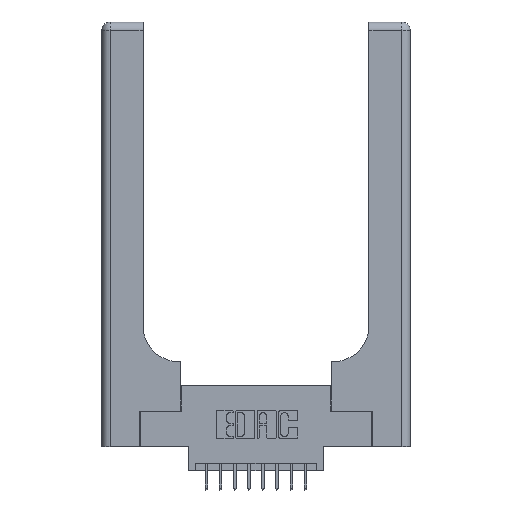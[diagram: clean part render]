
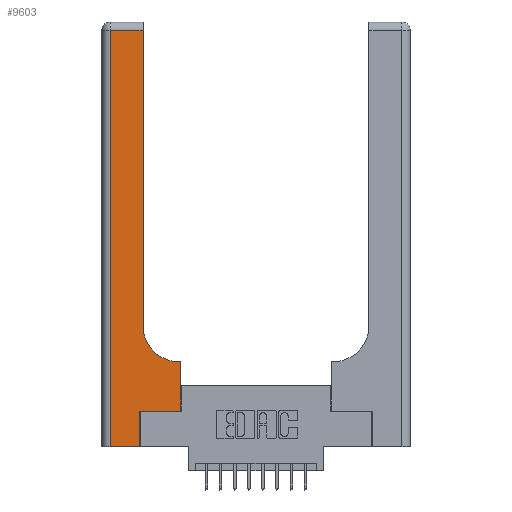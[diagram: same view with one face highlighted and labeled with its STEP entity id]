
A CAD part, top view. The second image highlights one B-rep face of the part: STEP entity #9603.
In plain terms, the highlighted planar face has unit normal (0, 0, 1).
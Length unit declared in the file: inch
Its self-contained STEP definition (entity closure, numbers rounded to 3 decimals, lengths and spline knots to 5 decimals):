
#223 = CARTESIAN_POINT ( 'NONE',  ( 0.2915, 2.94, 0.37 ) ) ;
#369 = DIRECTION ( 'NONE',  ( -1., 0., 0. ) ) ;
#524 = VERTEX_POINT ( 'NONE', #11892 ) ;
#541 = CARTESIAN_POINT ( 'NONE',  ( 0.2915, 3., 0.37 ) ) ;
#548 = CARTESIAN_POINT ( 'NONE',  ( 0.5415, 0.6, 0.37 ) ) ;
#1039 = ORIENTED_EDGE ( 'NONE', *, *, #4788, .T. ) ;
#1238 = VERTEX_POINT ( 'NONE', #223 ) ;
#1439 = CARTESIAN_POINT ( 'NONE',  ( 0., 2.94, 0.37 ) ) ;
#1464 = VERTEX_POINT ( 'NONE', #9798 ) ;
#1492 = AXIS2_PLACEMENT_3D ( 'NONE', #4526, #3270, #8075 ) ;
#1520 = LINE ( 'NONE', #5147, #5695 ) ;
#1839 = DIRECTION ( 'NONE',  ( -1., 0., 0. ) ) ;
#2392 = CARTESIAN_POINT ( 'NONE',  ( 0.06, 3., 0.37 ) ) ;
#2693 = DIRECTION ( 'NONE',  ( 0., 1., 0. ) ) ;
#2782 = ORIENTED_EDGE ( 'NONE', *, *, #4638, .T. ) ;
#2854 = VECTOR ( 'NONE', #6814, 39.37008 ) ;
#2928 = EDGE_CURVE ( 'NONE', #14129, #7966, #8968, .T. ) ;
#3190 = ORIENTED_EDGE ( 'NONE', *, *, #11571, .T. ) ;
#3215 = CARTESIAN_POINT ( 'NONE',  ( 0.269, 0.25, 0.37 ) ) ;
#3270 = DIRECTION ( 'NONE',  ( 0., 0., -1. ) ) ;
#3333 = ORIENTED_EDGE ( 'NONE', *, *, #12594, .T. ) ;
#3641 = EDGE_CURVE ( 'NONE', #1464, #1238, #4170, .T. ) ;
#3758 = CARTESIAN_POINT ( 'NONE',  ( 0.06, 2.94, 0.37 ) ) ;
#3923 = DIRECTION ( 'NONE',  ( -1., 0., 0. ) ) ;
#3999 = LINE ( 'NONE', #1439, #8890 ) ;
#4091 = CARTESIAN_POINT ( 'NONE',  ( 0.5585, 0.25, 0.37 ) ) ;
#4170 = LINE ( 'NONE', #541, #2854 ) ;
#4375 = CARTESIAN_POINT ( 'NONE',  ( 0.2915, 0.6, 0.37 ) ) ;
#4526 = CARTESIAN_POINT ( 'NONE',  ( 0.5415, 0.85, 0.37 ) ) ;
#4638 = EDGE_CURVE ( 'NONE', #10587, #1464, #10687, .T. ) ;
#4788 = EDGE_CURVE ( 'NONE', #15044, #14129, #1520, .T. ) ;
#4975 = CARTESIAN_POINT ( 'NONE',  ( 0.269, 0., 0.37 ) ) ;
#5147 = CARTESIAN_POINT ( 'NONE',  ( 0., 0., 0.37 ) ) ;
#5411 = VECTOR ( 'NONE', #11277, 39.37008 ) ;
#5695 = VECTOR ( 'NONE', #15281, 39.37008 ) ;
#6079 = VERTEX_POINT ( 'NONE', #3758 ) ;
#6111 = CARTESIAN_POINT ( 'NONE',  ( 0.269, 0.25, 0.37 ) ) ;
#6311 = CARTESIAN_POINT ( 'NONE',  ( 0.5585, 0.25, 0.37 ) ) ;
#6644 = FACE_OUTER_BOUND ( 'NONE', #7643, .T. ) ;
#6814 = DIRECTION ( 'NONE',  ( 0., 1., 0. ) ) ;
#7643 = EDGE_LOOP ( 'NONE', ( #9499, #9188, #3333, #1039, #12235, #13364, #3190, #9323, #2782 ) ) ;
#7966 = VERTEX_POINT ( 'NONE', #6111 ) ;
#7977 = AXIS2_PLACEMENT_3D ( 'NONE', #12908, #10178, #369 ) ;
#8075 = DIRECTION ( 'NONE',  ( 1., 0., 0. ) ) ;
#8827 = LINE ( 'NONE', #2392, #5411 ) ;
#8890 = VECTOR ( 'NONE', #3923, 39.37008 ) ;
#8968 = LINE ( 'NONE', #14131, #12256 ) ;
#8980 = LINE ( 'NONE', #4091, #15140 ) ;
#9188 = ORIENTED_EDGE ( 'NONE', *, *, #12989, .T. ) ;
#9323 = ORIENTED_EDGE ( 'NONE', *, *, #10077, .T. ) ;
#9499 = ORIENTED_EDGE ( 'NONE', *, *, #3641, .T. ) ;
#9603 = ADVANCED_FACE ( 'NONE', ( #6644 ), #14313, .F. ) ;
#9798 = CARTESIAN_POINT ( 'NONE',  ( 0.2915, 0.85, 0.37 ) ) ;
#10077 = EDGE_CURVE ( 'NONE', #524, #10587, #14097, .T. ) ;
#10178 = DIRECTION ( 'NONE',  ( 0., 0., -1. ) ) ;
#10587 = VERTEX_POINT ( 'NONE', #548 ) ;
#10687 = CIRCLE ( 'NONE', #1492, 0.25 ) ;
#11277 = DIRECTION ( 'NONE',  ( 0., -1., 0. ) ) ;
#11571 = EDGE_CURVE ( 'NONE', #15572, #524, #8980, .T. ) ;
#11892 = CARTESIAN_POINT ( 'NONE',  ( 0.5585, 0.6, 0.37 ) ) ;
#12235 = ORIENTED_EDGE ( 'NONE', *, *, #2928, .T. ) ;
#12256 = VECTOR ( 'NONE', #2693, 39.37008 ) ;
#12594 = EDGE_CURVE ( 'NONE', #6079, #15044, #8827, .T. ) ;
#12815 = VECTOR ( 'NONE', #13240, 39.37008 ) ;
#12908 = CARTESIAN_POINT ( 'NONE',  ( 0., 3., 0.37 ) ) ;
#12989 = EDGE_CURVE ( 'NONE', #1238, #6079, #3999, .T. ) ;
#13240 = DIRECTION ( 'NONE',  ( 1., 0., 0. ) ) ;
#13364 = ORIENTED_EDGE ( 'NONE', *, *, #13469, .T. ) ;
#13469 = EDGE_CURVE ( 'NONE', #7966, #15572, #14498, .T. ) ;
#13677 = CARTESIAN_POINT ( 'NONE',  ( 0.06, 0., 0.37 ) ) ;
#13939 = VECTOR ( 'NONE', #1839, 39.37008 ) ;
#13980 = DIRECTION ( 'NONE',  ( 0., 1., 0. ) ) ;
#14097 = LINE ( 'NONE', #4375, #13939 ) ;
#14129 = VERTEX_POINT ( 'NONE', #4975 ) ;
#14131 = CARTESIAN_POINT ( 'NONE',  ( 0.269, 0., 0.37 ) ) ;
#14313 = PLANE ( 'NONE',  #7977 ) ;
#14498 = LINE ( 'NONE', #3215, #12815 ) ;
#15044 = VERTEX_POINT ( 'NONE', #13677 ) ;
#15140 = VECTOR ( 'NONE', #13980, 39.37008 ) ;
#15281 = DIRECTION ( 'NONE',  ( 1., 0., 0. ) ) ;
#15572 = VERTEX_POINT ( 'NONE', #6311 ) ;
